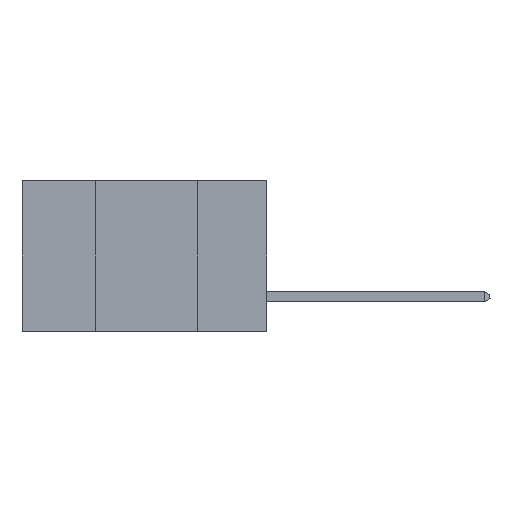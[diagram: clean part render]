
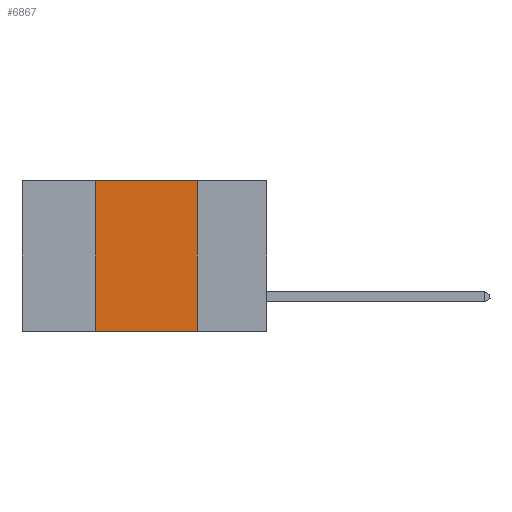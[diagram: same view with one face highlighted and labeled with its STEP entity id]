
A CAD part, left-side view. The second image highlights one B-rep face of the part: STEP entity #6867.
In plain terms, the highlighted planar face has unit normal (-1, 0, 0).
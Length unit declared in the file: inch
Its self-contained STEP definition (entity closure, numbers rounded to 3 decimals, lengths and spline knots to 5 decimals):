
#4553 = CARTESIAN_POINT ( 'NONE',  ( 0., 0.6, -0.37 ) ) ;
#4932 = DIRECTION ( 'NONE',  ( 0., 0., 1. ) ) ;
#5135 = DIRECTION ( 'NONE',  ( 0., -1., 0. ) ) ;
#5756 = FACE_OUTER_BOUND ( 'NONE', #26099, .T. ) ;
#6264 = CARTESIAN_POINT ( 'NONE',  ( 0., 0.6, 0. ) ) ;
#6867 = ADVANCED_FACE ( 'NONE', ( #5756 ), #8534, .F. ) ;
#7128 = CARTESIAN_POINT ( 'NONE',  ( 0., 0.17, 0. ) ) ;
#7612 = VECTOR ( 'NONE', #4932, 39.37008 ) ;
#7933 = EDGE_CURVE ( 'NONE', #16949, #13916, #12998, .T. ) ;
#8138 = EDGE_CURVE ( 'NONE', #8728, #13916, #11671, .T. ) ;
#8534 = PLANE ( 'NONE',  #18528 ) ;
#8728 = VERTEX_POINT ( 'NONE', #18395 ) ;
#8785 = DIRECTION ( 'NONE',  ( 0., -1., 0. ) ) ;
#9830 = CARTESIAN_POINT ( 'NONE',  ( 0., 0.42, -0.37 ) ) ;
#10604 = CARTESIAN_POINT ( 'NONE',  ( 0., 0.42, 0. ) ) ;
#11510 = DIRECTION ( 'NONE',  ( 0., 0., -1. ) ) ;
#11605 = CARTESIAN_POINT ( 'NONE',  ( 0., 0.6, 0. ) ) ;
#11671 = LINE ( 'NONE', #7128, #19608 ) ;
#11978 = ORIENTED_EDGE ( 'NONE', *, *, #8138, .F. ) ;
#12998 = LINE ( 'NONE', #4553, #23939 ) ;
#13916 = VERTEX_POINT ( 'NONE', #19361 ) ;
#14088 = VECTOR ( 'NONE', #5135, 39.37008 ) ;
#14974 = DIRECTION ( 'NONE',  ( 0., 0., -1. ) ) ;
#16746 = EDGE_CURVE ( 'NONE', #24260, #8728, #24627, .T. ) ;
#16949 = VERTEX_POINT ( 'NONE', #9830 ) ;
#17611 = ORIENTED_EDGE ( 'NONE', *, *, #16746, .F. ) ;
#18395 = CARTESIAN_POINT ( 'NONE',  ( 0., 0.17, 0. ) ) ;
#18528 = AXIS2_PLACEMENT_3D ( 'NONE', #6264, #19215, #14974 ) ;
#18572 = LINE ( 'NONE', #26029, #7612 ) ;
#19213 = EDGE_CURVE ( 'NONE', #16949, #24260, #18572, .T. ) ;
#19215 = DIRECTION ( 'NONE',  ( 1., 0., 0. ) ) ;
#19361 = CARTESIAN_POINT ( 'NONE',  ( 0., 0.17, -0.37 ) ) ;
#19608 = VECTOR ( 'NONE', #11510, 39.37008 ) ;
#23939 = VECTOR ( 'NONE', #8785, 39.37008 ) ;
#24260 = VERTEX_POINT ( 'NONE', #10604 ) ;
#24627 = LINE ( 'NONE', #11605, #14088 ) ;
#25858 = ORIENTED_EDGE ( 'NONE', *, *, #7933, .T. ) ;
#26029 = CARTESIAN_POINT ( 'NONE',  ( 0., 0.42, 0. ) ) ;
#26099 = EDGE_LOOP ( 'NONE', ( #11978, #17611, #26114, #25858 ) ) ;
#26114 = ORIENTED_EDGE ( 'NONE', *, *, #19213, .F. ) ;
